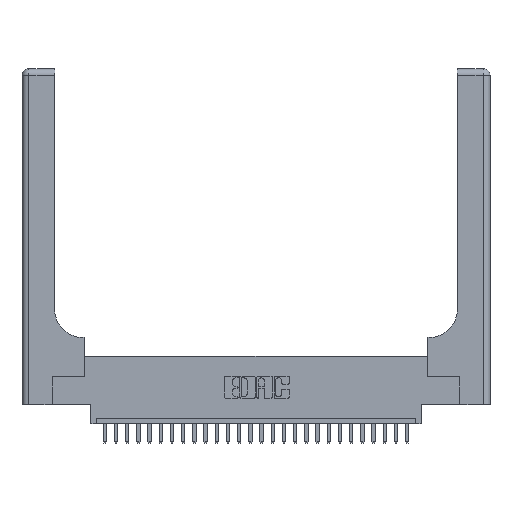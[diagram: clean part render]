
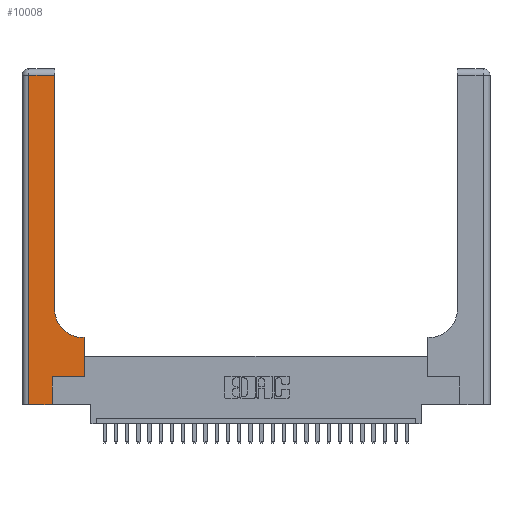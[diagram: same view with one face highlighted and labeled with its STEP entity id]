
A CAD part, top view. The second image highlights one B-rep face of the part: STEP entity #10008.
In plain terms, the highlighted planar face has unit normal (0, 0, 1).
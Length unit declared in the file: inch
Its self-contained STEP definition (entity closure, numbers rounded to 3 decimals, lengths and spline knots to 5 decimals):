
#305 = VERTEX_POINT ( 'NONE', #6612 ) ;
#526 = LINE ( 'NONE', #28338, #8430 ) ;
#747 = EDGE_CURVE ( 'NONE', #5410, #25173, #26032, .T. ) ;
#791 = CARTESIAN_POINT ( 'NONE',  ( 0., 2.94, 0.37 ) ) ;
#886 = DIRECTION ( 'NONE',  ( -1., 0., 0. ) ) ;
#1436 = AXIS2_PLACEMENT_3D ( 'NONE', #5959, #25594, #8149 ) ;
#1470 = PLANE ( 'NONE',  #23376 ) ;
#2207 = EDGE_CURVE ( 'NONE', #19924, #14634, #6731, .T. ) ;
#2228 = VECTOR ( 'NONE', #5100, 39.37008 ) ;
#3372 = DIRECTION ( 'NONE',  ( -1., 0., 0. ) ) ;
#4876 = FACE_OUTER_BOUND ( 'NONE', #19764, .T. ) ;
#5100 = DIRECTION ( 'NONE',  ( 1., 0., 0. ) ) ;
#5410 = VERTEX_POINT ( 'NONE', #7674 ) ;
#5959 = CARTESIAN_POINT ( 'NONE',  ( 0.5415, 0.85, 0.37 ) ) ;
#6494 = ORIENTED_EDGE ( 'NONE', *, *, #25731, .T. ) ;
#6612 = CARTESIAN_POINT ( 'NONE',  ( 0.269, 0.25, 0.37 ) ) ;
#6731 = LINE ( 'NONE', #27882, #18089 ) ;
#6869 = VERTEX_POINT ( 'NONE', #27940 ) ;
#6963 = EDGE_CURVE ( 'NONE', #21170, #19924, #16000, .T. ) ;
#7133 = CARTESIAN_POINT ( 'NONE',  ( 0., 0., 0.37 ) ) ;
#7219 = EDGE_CURVE ( 'NONE', #19438, #21170, #15975, .T. ) ;
#7557 = VECTOR ( 'NONE', #12065, 39.37008 ) ;
#7674 = CARTESIAN_POINT ( 'NONE',  ( 0.5585, 0.25, 0.37 ) ) ;
#8094 = VERTEX_POINT ( 'NONE', #15920 ) ;
#8149 = DIRECTION ( 'NONE',  ( 1., 0., 0. ) ) ;
#8430 = VECTOR ( 'NONE', #12744, 39.37008 ) ;
#9109 = CARTESIAN_POINT ( 'NONE',  ( 0.5585, 0.25, 0.37 ) ) ;
#9294 = DIRECTION ( 'NONE',  ( 0., 1., 0. ) ) ;
#9669 = CARTESIAN_POINT ( 'NONE',  ( 0.2915, 0.85, 0.37 ) ) ;
#9848 = CARTESIAN_POINT ( 'NONE',  ( 0.269, 0., 0.37 ) ) ;
#10008 = ADVANCED_FACE ( 'NONE', ( #4876 ), #1470, .F. ) ;
#11320 = ORIENTED_EDGE ( 'NONE', *, *, #27057, .T. ) ;
#11798 = DIRECTION ( 'NONE',  ( 1., 0., 0. ) ) ;
#12060 = ORIENTED_EDGE ( 'NONE', *, *, #2207, .T. ) ;
#12065 = DIRECTION ( 'NONE',  ( 0., 1., 0. ) ) ;
#12200 = CARTESIAN_POINT ( 'NONE',  ( 0., 3., 0.37 ) ) ;
#12744 = DIRECTION ( 'NONE',  ( -1., 0., 0. ) ) ;
#13330 = VECTOR ( 'NONE', #9294, 39.37008 ) ;
#13404 = EDGE_CURVE ( 'NONE', #6869, #305, #16796, .T. ) ;
#14634 = VERTEX_POINT ( 'NONE', #28210 ) ;
#14756 = DIRECTION ( 'NONE',  ( 0., -1., 0. ) ) ;
#15459 = ORIENTED_EDGE ( 'NONE', *, *, #27341, .T. ) ;
#15920 = CARTESIAN_POINT ( 'NONE',  ( 0.5415, 0.6, 0.37 ) ) ;
#15975 = LINE ( 'NONE', #23002, #17028 ) ;
#16000 = LINE ( 'NONE', #791, #25947 ) ;
#16510 = DIRECTION ( 'NONE',  ( 0., 1., 0. ) ) ;
#16794 = DIRECTION ( 'NONE',  ( 0., 0., -1. ) ) ;
#16796 = LINE ( 'NONE', #9848, #7557 ) ;
#17028 = VECTOR ( 'NONE', #16510, 39.37008 ) ;
#17398 = LINE ( 'NONE', #18418, #20457 ) ;
#18089 = VECTOR ( 'NONE', #14756, 39.37008 ) ;
#18418 = CARTESIAN_POINT ( 'NONE',  ( 0.269, 0.25, 0.37 ) ) ;
#18751 = ORIENTED_EDGE ( 'NONE', *, *, #28178, .T. ) ;
#19438 = VERTEX_POINT ( 'NONE', #9669 ) ;
#19501 = ORIENTED_EDGE ( 'NONE', *, *, #6963, .T. ) ;
#19764 = EDGE_LOOP ( 'NONE', ( #20744, #19501, #12060, #18751, #21586, #11320, #23469, #15459, #6494 ) ) ;
#19924 = VERTEX_POINT ( 'NONE', #22756 ) ;
#20300 = CIRCLE ( 'NONE', #1436, 0.25 ) ;
#20457 = VECTOR ( 'NONE', #11798, 39.37008 ) ;
#20720 = CARTESIAN_POINT ( 'NONE',  ( 0.2915, 2.94, 0.37 ) ) ;
#20744 = ORIENTED_EDGE ( 'NONE', *, *, #7219, .T. ) ;
#21035 = CARTESIAN_POINT ( 'NONE',  ( 0.5585, 0.6, 0.37 ) ) ;
#21170 = VERTEX_POINT ( 'NONE', #20720 ) ;
#21586 = ORIENTED_EDGE ( 'NONE', *, *, #13404, .T. ) ;
#22756 = CARTESIAN_POINT ( 'NONE',  ( 0.06, 2.94, 0.37 ) ) ;
#23002 = CARTESIAN_POINT ( 'NONE',  ( 0.2915, 3., 0.37 ) ) ;
#23376 = AXIS2_PLACEMENT_3D ( 'NONE', #12200, #16794, #3372 ) ;
#23469 = ORIENTED_EDGE ( 'NONE', *, *, #747, .T. ) ;
#24168 = LINE ( 'NONE', #7133, #2228 ) ;
#25173 = VERTEX_POINT ( 'NONE', #21035 ) ;
#25594 = DIRECTION ( 'NONE',  ( 0., 0., -1. ) ) ;
#25731 = EDGE_CURVE ( 'NONE', #8094, #19438, #20300, .T. ) ;
#25947 = VECTOR ( 'NONE', #886, 39.37008 ) ;
#26032 = LINE ( 'NONE', #9109, #13330 ) ;
#27057 = EDGE_CURVE ( 'NONE', #305, #5410, #17398, .T. ) ;
#27341 = EDGE_CURVE ( 'NONE', #25173, #8094, #526, .T. ) ;
#27882 = CARTESIAN_POINT ( 'NONE',  ( 0.06, 3., 0.37 ) ) ;
#27940 = CARTESIAN_POINT ( 'NONE',  ( 0.269, 0., 0.37 ) ) ;
#28178 = EDGE_CURVE ( 'NONE', #14634, #6869, #24168, .T. ) ;
#28210 = CARTESIAN_POINT ( 'NONE',  ( 0.06, 0., 0.37 ) ) ;
#28338 = CARTESIAN_POINT ( 'NONE',  ( 0.2915, 0.6, 0.37 ) ) ;
